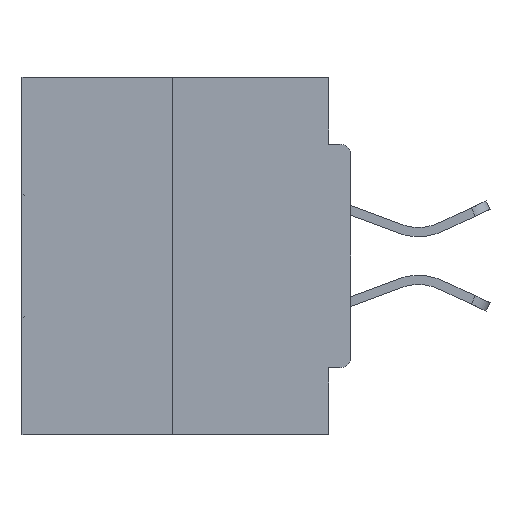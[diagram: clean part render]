
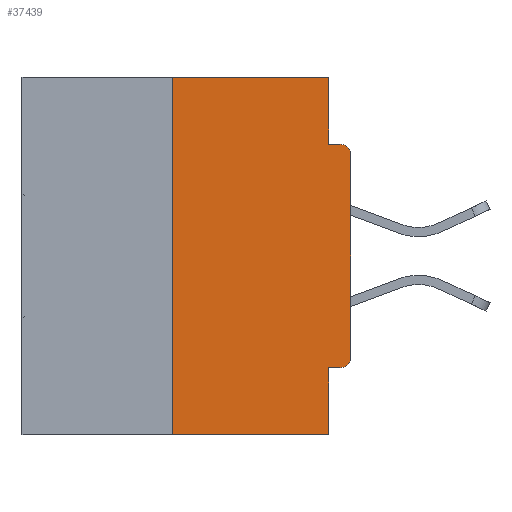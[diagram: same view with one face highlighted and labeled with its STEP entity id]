
A CAD part, left-side view. The second image highlights one B-rep face of the part: STEP entity #37439.
In plain terms, the highlighted planar face has unit normal (-1, 0, 0).
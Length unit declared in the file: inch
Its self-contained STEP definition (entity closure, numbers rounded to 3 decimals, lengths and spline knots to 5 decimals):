
#410 = CARTESIAN_POINT ( 'NONE',  ( 0., 0.031, -0.5 ) ) ;
#775 = VERTEX_POINT ( 'NONE', #7501 ) ;
#1146 = CIRCLE ( 'NONE', #37501, 0.015 ) ;
#1250 = VERTEX_POINT ( 'NONE', #29032 ) ;
#1454 = DIRECTION ( 'NONE',  ( 0., -1., 0. ) ) ;
#1616 = EDGE_CURVE ( 'NONE', #18556, #8102, #9572, .T. ) ;
#1943 = ORIENTED_EDGE ( 'NONE', *, *, #25215, .T. ) ;
#2343 = CARTESIAN_POINT ( 'NONE',  ( 0., 0.46, 0. ) ) ;
#2413 = CARTESIAN_POINT ( 'NONE',  ( 0., 0.25, 0. ) ) ;
#3548 = DIRECTION ( 'NONE',  ( 0., -1., 0. ) ) ;
#3599 = LINE ( 'NONE', #20854, #5540 ) ;
#5540 = VECTOR ( 'NONE', #27171, 39.37008 ) ;
#6509 = AXIS2_PLACEMENT_3D ( 'NONE', #16573, #32227, #25495 ) ;
#6645 = DIRECTION ( 'NONE',  ( 0., 0., -1. ) ) ;
#7154 = VERTEX_POINT ( 'NONE', #25097 ) ;
#7501 = CARTESIAN_POINT ( 'NONE',  ( 0., 0.25, -0.5 ) ) ;
#8102 = VERTEX_POINT ( 'NONE', #9482 ) ;
#8775 = CIRCLE ( 'NONE', #6509, 0.015 ) ;
#9482 = CARTESIAN_POINT ( 'NONE',  ( 0., 0.031, -0.4065 ) ) ;
#9572 = LINE ( 'NONE', #18270, #19137 ) ;
#10292 = LINE ( 'NONE', #30914, #37767 ) ;
#10391 = EDGE_CURVE ( 'NONE', #1250, #26287, #24678, .T. ) ;
#11190 = ORIENTED_EDGE ( 'NONE', *, *, #1616, .F. ) ;
#11835 = DIRECTION ( 'NONE',  ( 0., 0., -1. ) ) ;
#13608 = VECTOR ( 'NONE', #33083, 39.37008 ) ;
#13718 = CARTESIAN_POINT ( 'NONE',  ( 0., 0., -0.0935 ) ) ;
#13719 = DIRECTION ( 'NONE',  ( 0., 0., -1. ) ) ;
#14488 = ORIENTED_EDGE ( 'NONE', *, *, #30507, .F. ) ;
#14538 = EDGE_CURVE ( 'NONE', #7154, #33436, #1146, .T. ) ;
#14719 = EDGE_LOOP ( 'NONE', ( #38813, #14488, #27719, #20962, #11190, #1943, #38459, #19715, #15692, #18807 ) ) ;
#15133 = DIRECTION ( 'NONE',  ( 0., -1., 0. ) ) ;
#15295 = CARTESIAN_POINT ( 'NONE',  ( 0., 0.46, 0. ) ) ;
#15692 = ORIENTED_EDGE ( 'NONE', *, *, #25818, .F. ) ;
#15886 = VECTOR ( 'NONE', #1454, 39.37008 ) ;
#16573 = CARTESIAN_POINT ( 'NONE',  ( 0., 0.015, -0.3915 ) ) ;
#17240 = LINE ( 'NONE', #410, #27380 ) ;
#17384 = EDGE_CURVE ( 'NONE', #22071, #1250, #38046, .T. ) ;
#18270 = CARTESIAN_POINT ( 'NONE',  ( 0., 0., -0.4065 ) ) ;
#18340 = LINE ( 'NONE', #2413, #13608 ) ;
#18556 = VERTEX_POINT ( 'NONE', #33880 ) ;
#18807 = ORIENTED_EDGE ( 'NONE', *, *, #10391, .F. ) ;
#19127 = EDGE_CURVE ( 'NONE', #8102, #33636, #17240, .T. ) ;
#19137 = VECTOR ( 'NONE', #27578, 39.37008 ) ;
#19253 = LINE ( 'NONE', #13718, #15886 ) ;
#19715 = ORIENTED_EDGE ( 'NONE', *, *, #14538, .T. ) ;
#20332 = PLANE ( 'NONE',  #37594 ) ;
#20650 = DIRECTION ( 'NONE',  ( -1., 0., 0. ) ) ;
#20854 = CARTESIAN_POINT ( 'NONE',  ( 0., 0., 0. ) ) ;
#20962 = ORIENTED_EDGE ( 'NONE', *, *, #19127, .F. ) ;
#22071 = VERTEX_POINT ( 'NONE', #38951 ) ;
#22669 = CARTESIAN_POINT ( 'NONE',  ( 0., 0.031, -0.5 ) ) ;
#24678 = LINE ( 'NONE', #28891, #38763 ) ;
#25097 = CARTESIAN_POINT ( 'NONE',  ( 0., 0., -0.1085 ) ) ;
#25215 = EDGE_CURVE ( 'NONE', #18556, #26568, #8775, .T. ) ;
#25495 = DIRECTION ( 'NONE',  ( 0., 0., -1. ) ) ;
#25818 = EDGE_CURVE ( 'NONE', #26287, #33436, #19253, .T. ) ;
#26287 = VERTEX_POINT ( 'NONE', #39243 ) ;
#26393 = DIRECTION ( 'NONE',  ( 0., 0., -1. ) ) ;
#26568 = VERTEX_POINT ( 'NONE', #39288 ) ;
#27171 = DIRECTION ( 'NONE',  ( 0., 0., 1. ) ) ;
#27380 = VECTOR ( 'NONE', #6645, 39.37008 ) ;
#27578 = DIRECTION ( 'NONE',  ( 0., 1., 0. ) ) ;
#27719 = ORIENTED_EDGE ( 'NONE', *, *, #34198, .T. ) ;
#28308 = VECTOR ( 'NONE', #3548, 39.37008 ) ;
#28891 = CARTESIAN_POINT ( 'NONE',  ( 0., 0.031, 0. ) ) ;
#29032 = CARTESIAN_POINT ( 'NONE',  ( 0., 0.031, 0. ) ) ;
#30507 = EDGE_CURVE ( 'NONE', #775, #22071, #18340, .T. ) ;
#30914 = CARTESIAN_POINT ( 'NONE',  ( 0., 0.46, -0.5 ) ) ;
#32227 = DIRECTION ( 'NONE',  ( -1., 0., 0. ) ) ;
#32474 = DIRECTION ( 'NONE',  ( 1., 0., 0. ) ) ;
#33083 = DIRECTION ( 'NONE',  ( 0., 0., 1. ) ) ;
#33436 = VERTEX_POINT ( 'NONE', #39774 ) ;
#33636 = VERTEX_POINT ( 'NONE', #22669 ) ;
#33880 = CARTESIAN_POINT ( 'NONE',  ( 0., 0.015, -0.4065 ) ) ;
#34198 = EDGE_CURVE ( 'NONE', #775, #33636, #10292, .T. ) ;
#35293 = FACE_OUTER_BOUND ( 'NONE', #14719, .T. ) ;
#36220 = CARTESIAN_POINT ( 'NONE',  ( 0., 0.015, -0.1085 ) ) ;
#37439 = ADVANCED_FACE ( 'NONE', ( #35293 ), #20332, .F. ) ;
#37501 = AXIS2_PLACEMENT_3D ( 'NONE', #36220, #20650, #11835 ) ;
#37594 = AXIS2_PLACEMENT_3D ( 'NONE', #2343, #32474, #26393 ) ;
#37767 = VECTOR ( 'NONE', #15133, 39.37008 ) ;
#38046 = LINE ( 'NONE', #15295, #28308 ) ;
#38459 = ORIENTED_EDGE ( 'NONE', *, *, #39664, .T. ) ;
#38763 = VECTOR ( 'NONE', #13719, 39.37008 ) ;
#38813 = ORIENTED_EDGE ( 'NONE', *, *, #17384, .F. ) ;
#38951 = CARTESIAN_POINT ( 'NONE',  ( 0., 0.25, 0. ) ) ;
#39243 = CARTESIAN_POINT ( 'NONE',  ( 0., 0.031, -0.0935 ) ) ;
#39288 = CARTESIAN_POINT ( 'NONE',  ( 0., 0., -0.3915 ) ) ;
#39664 = EDGE_CURVE ( 'NONE', #26568, #7154, #3599, .T. ) ;
#39774 = CARTESIAN_POINT ( 'NONE',  ( 0., 0.015, -0.0935 ) ) ;
